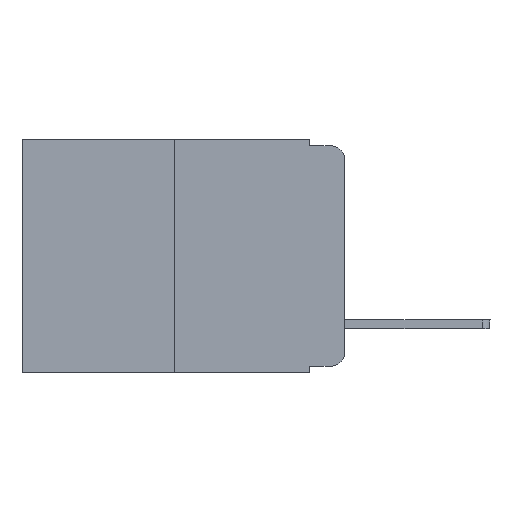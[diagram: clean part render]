
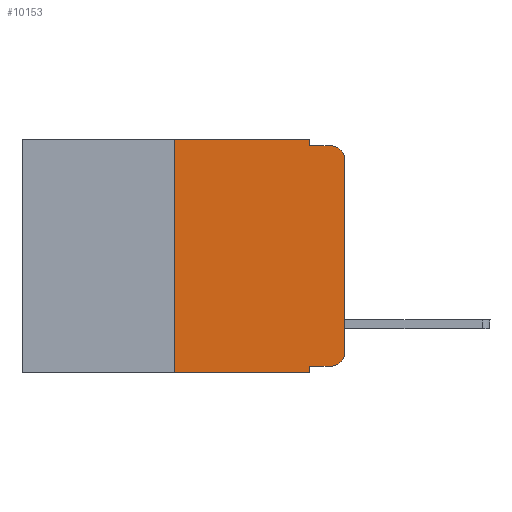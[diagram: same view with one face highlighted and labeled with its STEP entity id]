
A CAD part, left-side view. The second image highlights one B-rep face of the part: STEP entity #10153.
In plain terms, the highlighted planar face has unit normal (-1, 0, 0).
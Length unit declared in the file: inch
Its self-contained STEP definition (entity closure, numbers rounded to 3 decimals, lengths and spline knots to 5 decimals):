
#193 = DIRECTION ( 'NONE',  ( 0., -1., 0. ) ) ;
#454 = CARTESIAN_POINT ( 'NONE',  ( 0., 0.25, 0. ) ) ;
#625 = VERTEX_POINT ( 'NONE', #454 ) ;
#704 = ORIENTED_EDGE ( 'NONE', *, *, #1044, .T. ) ;
#1044 = EDGE_CURVE ( 'NONE', #20722, #15848, #1333, .T. ) ;
#1333 = CIRCLE ( 'NONE', #2809, 0.02 ) ;
#1441 = EDGE_LOOP ( 'NONE', ( #15006, #704, #12803, #5872, #22608, #4568, #20913, #8392, #17904, #18496 ) ) ;
#1463 = VECTOR ( 'NONE', #10822, 39.37008 ) ;
#1934 = VERTEX_POINT ( 'NONE', #6519 ) ;
#2292 = CARTESIAN_POINT ( 'NONE',  ( 0., 0.02, -0.313 ) ) ;
#2310 = LINE ( 'NONE', #11095, #19515 ) ;
#2323 = DIRECTION ( 'NONE',  ( 0., 0., -1. ) ) ;
#2809 = AXIS2_PLACEMENT_3D ( 'NONE', #18412, #18523, #2323 ) ;
#3291 = VERTEX_POINT ( 'NONE', #7933 ) ;
#3406 = VECTOR ( 'NONE', #10807, 39.37008 ) ;
#3570 = CARTESIAN_POINT ( 'NONE',  ( 0., 0.25, 0. ) ) ;
#3653 = LINE ( 'NONE', #12596, #1463 ) ;
#3975 = DIRECTION ( 'NONE',  ( 0., 0., -1. ) ) ;
#4148 = CARTESIAN_POINT ( 'NONE',  ( 0., 0.25, -0.343 ) ) ;
#4383 = DIRECTION ( 'NONE',  ( 0., 0., -1. ) ) ;
#4449 = LINE ( 'NONE', #22190, #17911 ) ;
#4568 = ORIENTED_EDGE ( 'NONE', *, *, #5472, .F. ) ;
#4940 = CARTESIAN_POINT ( 'NONE',  ( 0., 0.473, 0. ) ) ;
#5472 = EDGE_CURVE ( 'NONE', #19431, #625, #8893, .T. ) ;
#5631 = LINE ( 'NONE', #10777, #20204 ) ;
#5872 = ORIENTED_EDGE ( 'NONE', *, *, #17655, .F. ) ;
#6519 = CARTESIAN_POINT ( 'NONE',  ( 0., 0.02, -0.333 ) ) ;
#6795 = EDGE_CURVE ( 'NONE', #625, #14792, #14935, .T. ) ;
#7005 = VERTEX_POINT ( 'NONE', #18086 ) ;
#7171 = DIRECTION ( 'NONE',  ( 0., -1., 0. ) ) ;
#7428 = EDGE_CURVE ( 'NONE', #22931, #1934, #21819, .T. ) ;
#7524 = CARTESIAN_POINT ( 'NONE',  ( 0., 0.02, -0.01 ) ) ;
#7933 = CARTESIAN_POINT ( 'NONE',  ( 0., 0.051, -0.01 ) ) ;
#8392 = ORIENTED_EDGE ( 'NONE', *, *, #10158, .F. ) ;
#8406 = CARTESIAN_POINT ( 'NONE',  ( 0., 0.051, 0. ) ) ;
#8893 = LINE ( 'NONE', #3570, #19041 ) ;
#8935 = VERTEX_POINT ( 'NONE', #15470 ) ;
#9443 = EDGE_CURVE ( 'NONE', #3291, #15848, #3653, .T. ) ;
#9566 = DIRECTION ( 'NONE',  ( -1., 0., 0. ) ) ;
#9729 = DIRECTION ( 'NONE',  ( 1., 0., 0. ) ) ;
#10153 = ADVANCED_FACE ( 'NONE', ( #22302 ), #11388, .F. ) ;
#10158 = EDGE_CURVE ( 'NONE', #22931, #8935, #4449, .T. ) ;
#10168 = CARTESIAN_POINT ( 'NONE',  ( 0., 0.051, -0.333 ) ) ;
#10409 = AXIS2_PLACEMENT_3D ( 'NONE', #2292, #9566, #4383 ) ;
#10777 = CARTESIAN_POINT ( 'NONE',  ( 0., 0.473, -0.343 ) ) ;
#10807 = DIRECTION ( 'NONE',  ( 0., 0., 1. ) ) ;
#10822 = DIRECTION ( 'NONE',  ( 0., -1., 0. ) ) ;
#11089 = DIRECTION ( 'NONE',  ( 0., 0., 1. ) ) ;
#11095 = CARTESIAN_POINT ( 'NONE',  ( 0., 0.051, 0. ) ) ;
#11159 = CIRCLE ( 'NONE', #10409, 0.02 ) ;
#11388 = PLANE ( 'NONE',  #20188 ) ;
#11504 = CARTESIAN_POINT ( 'NONE',  ( 0., 0.473, 0. ) ) ;
#12102 = DIRECTION ( 'NONE',  ( 0., -1., 0. ) ) ;
#12596 = CARTESIAN_POINT ( 'NONE',  ( 0., 0.051, -0.01 ) ) ;
#12803 = ORIENTED_EDGE ( 'NONE', *, *, #9443, .F. ) ;
#13447 = EDGE_CURVE ( 'NONE', #1934, #7005, #11159, .T. ) ;
#14792 = VERTEX_POINT ( 'NONE', #8406 ) ;
#14935 = LINE ( 'NONE', #4940, #18892 ) ;
#15006 = ORIENTED_EDGE ( 'NONE', *, *, #18407, .T. ) ;
#15470 = CARTESIAN_POINT ( 'NONE',  ( 0., 0.051, -0.343 ) ) ;
#15689 = EDGE_CURVE ( 'NONE', #19431, #8935, #5631, .T. ) ;
#15848 = VERTEX_POINT ( 'NONE', #7524 ) ;
#16718 = CARTESIAN_POINT ( 'NONE',  ( 0., 0., -0.03 ) ) ;
#17655 = EDGE_CURVE ( 'NONE', #14792, #3291, #2310, .T. ) ;
#17904 = ORIENTED_EDGE ( 'NONE', *, *, #7428, .T. ) ;
#17911 = VECTOR ( 'NONE', #3975, 39.37008 ) ;
#18086 = CARTESIAN_POINT ( 'NONE',  ( 0., 0., -0.313 ) ) ;
#18407 = EDGE_CURVE ( 'NONE', #7005, #20722, #22921, .T. ) ;
#18412 = CARTESIAN_POINT ( 'NONE',  ( 0., 0.02, -0.03 ) ) ;
#18496 = ORIENTED_EDGE ( 'NONE', *, *, #13447, .T. ) ;
#18523 = DIRECTION ( 'NONE',  ( -1., 0., 0. ) ) ;
#18650 = VECTOR ( 'NONE', #193, 39.37008 ) ;
#18777 = DIRECTION ( 'NONE',  ( 0., 0., -1. ) ) ;
#18892 = VECTOR ( 'NONE', #12102, 39.37008 ) ;
#19041 = VECTOR ( 'NONE', #11089, 39.37008 ) ;
#19431 = VERTEX_POINT ( 'NONE', #4148 ) ;
#19515 = VECTOR ( 'NONE', #21910, 39.37008 ) ;
#19706 = CARTESIAN_POINT ( 'NONE',  ( 0., 0.051, -0.333 ) ) ;
#19877 = CARTESIAN_POINT ( 'NONE',  ( 0., 0., 0. ) ) ;
#20188 = AXIS2_PLACEMENT_3D ( 'NONE', #11504, #9729, #18777 ) ;
#20204 = VECTOR ( 'NONE', #7171, 39.37008 ) ;
#20722 = VERTEX_POINT ( 'NONE', #16718 ) ;
#20913 = ORIENTED_EDGE ( 'NONE', *, *, #15689, .T. ) ;
#21819 = LINE ( 'NONE', #19706, #18650 ) ;
#21910 = DIRECTION ( 'NONE',  ( 0., 0., -1. ) ) ;
#22190 = CARTESIAN_POINT ( 'NONE',  ( 0., 0.051, 0. ) ) ;
#22302 = FACE_OUTER_BOUND ( 'NONE', #1441, .T. ) ;
#22608 = ORIENTED_EDGE ( 'NONE', *, *, #6795, .F. ) ;
#22921 = LINE ( 'NONE', #19877, #3406 ) ;
#22931 = VERTEX_POINT ( 'NONE', #10168 ) ;
